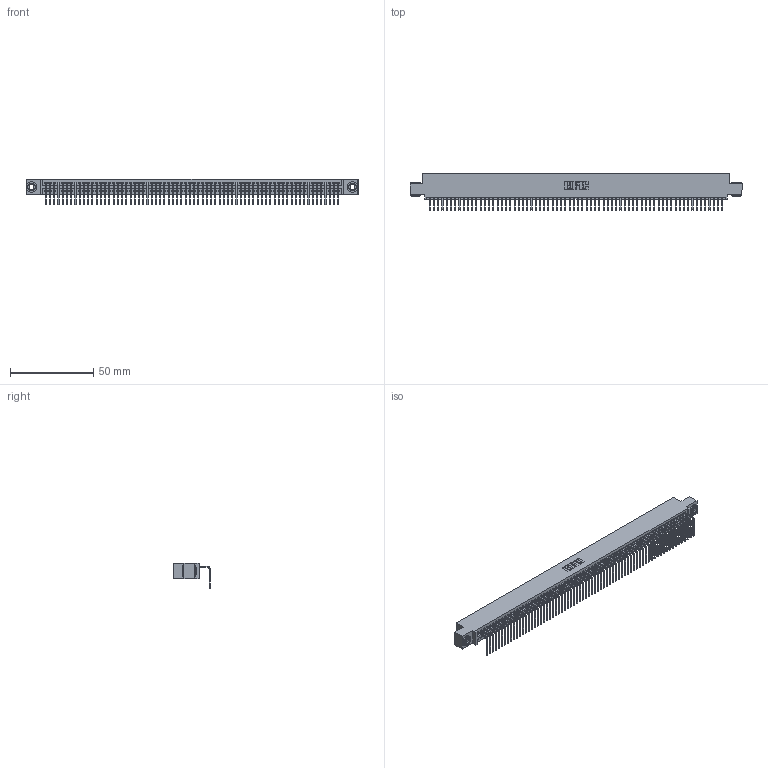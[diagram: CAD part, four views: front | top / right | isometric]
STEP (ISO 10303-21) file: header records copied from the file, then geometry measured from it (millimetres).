
FILE_DESCRIPTION (( 'STEP AP203' ), '1' );
FILE_NAME ('395-070-558-403.STEP', '2018-11-27T02:01:34', ( '' ), ( '' ), 'SwSTEP 2.0', 'SolidWorks 2016', '' );
FILE_SCHEMA (( 'CONFIG_CONTROL_DESIGN' ));
Length unit declared in the file: inch
Products named in the file (4): 395-070-558-403; 345 Part_0.110 Offset - 0.156 Dia-TH; 345-250-002_345-250-002-102; 345-292-001_558 Tail - 2
Assembly tree (73 placements, depth 2):
  395-070-558-403
    345 Part_0.110 Offset - 0.156 Dia-TH
    345-292-001_558 Tail - 2  x70
    345-250-002_345-250-002-102  x2
Bounding box: 199.01 x 21.83 x 15.37 mm (x, y, z)
Volume: 19310.7 mm3; surface area: 27709.5 mm2
Topology: 73 solids, 73 shells, 4368 faces, 13169 edges, 8682 vertices
Faces by surface type: plane 3034, cylinder 1326, cone 8
Entity records: 49780 total; most frequent: CARTESIAN_POINT 8601, ORIENTED_EDGE 8598, DIRECTION 7501, EDGE_CURVE 4299, VECTOR 3863, LINE 3863, VERTEX_POINT 2862, AXIS2_PLACEMENT_3D 1819
